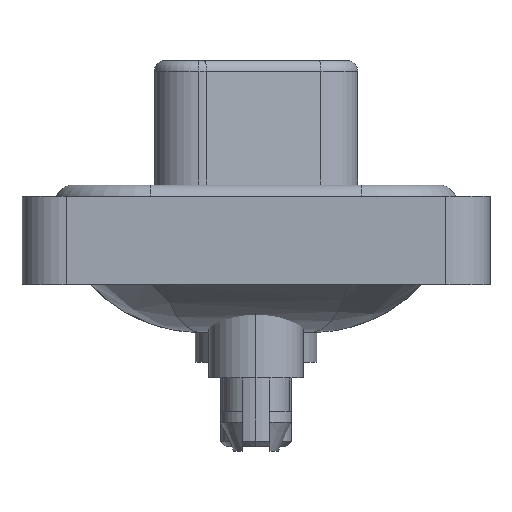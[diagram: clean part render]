
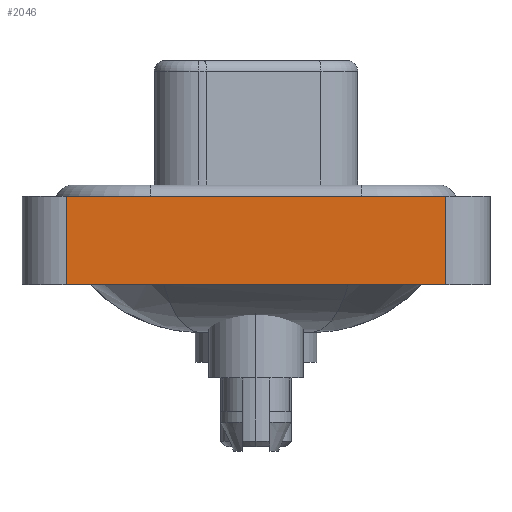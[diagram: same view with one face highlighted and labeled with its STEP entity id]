
A CAD part, left-side view. The second image highlights one B-rep face of the part: STEP entity #2046.
In plain terms, the highlighted planar face has unit normal (-1, 0, 0).
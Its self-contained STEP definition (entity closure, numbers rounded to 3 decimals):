
#1692 = DIRECTION ( 'NONE',  ( 0., -1., 0. ) ) ;
#2046 = ADVANCED_FACE ( 'NONE', ( #7169 ), #2827, .T. ) ;
#2258 = CARTESIAN_POINT ( 'NONE',  ( -7.25, -8.55, -3.6 ) ) ;
#2672 = LINE ( 'NONE', #9816, #17047 ) ;
#2827 = PLANE ( 'NONE',  #12891 ) ;
#2926 = DIRECTION ( 'NONE',  ( -1., 0., 0. ) ) ;
#3456 = VERTEX_POINT ( 'NONE', #10080 ) ;
#3554 = VERTEX_POINT ( 'NONE', #2258 ) ;
#3584 = VECTOR ( 'NONE', #5927, 1000. ) ;
#3691 = VECTOR ( 'NONE', #1692, 1000. ) ;
#3720 = EDGE_CURVE ( 'NONE', #3456, #3554, #6868, .T. ) ;
#4856 = ORIENTED_EDGE ( 'NONE', *, *, #5806, .F. ) ;
#5455 = CARTESIAN_POINT ( 'NONE',  ( -7.25, -8.55, -3.6 ) ) ;
#5572 = DIRECTION ( 'NONE',  ( 0., 0., 1. ) ) ;
#5806 = EDGE_CURVE ( 'NONE', #16466, #14909, #5889, .T. ) ;
#5889 = LINE ( 'NONE', #10043, #3691 ) ;
#5927 = DIRECTION ( 'NONE',  ( 0., 0., 1. ) ) ;
#6868 = LINE ( 'NONE', #5455, #8618 ) ;
#7169 = FACE_OUTER_BOUND ( 'NONE', #17721, .T. ) ;
#7409 = ORIENTED_EDGE ( 'NONE', *, *, #3720, .T. ) ;
#7937 = CARTESIAN_POINT ( 'NONE',  ( -7.25, -8.55, 0.4 ) ) ;
#8618 = VECTOR ( 'NONE', #9496, 1000. ) ;
#9496 = DIRECTION ( 'NONE',  ( 0., -1., 0. ) ) ;
#9816 = CARTESIAN_POINT ( 'NONE',  ( -7.25, -8.55, -3.6 ) ) ;
#9972 = EDGE_CURVE ( 'NONE', #3456, #16466, #15816, .T. ) ;
#10043 = CARTESIAN_POINT ( 'NONE',  ( -7.25, -8.55, 0.4 ) ) ;
#10080 = CARTESIAN_POINT ( 'NONE',  ( -7.25, 8.55, -3.6 ) ) ;
#12891 = AXIS2_PLACEMENT_3D ( 'NONE', #14225, #2926, #14500 ) ;
#13323 = ORIENTED_EDGE ( 'NONE', *, *, #9972, .F. ) ;
#14225 = CARTESIAN_POINT ( 'NONE',  ( -7.25, -8.55, -3.6 ) ) ;
#14500 = DIRECTION ( 'NONE',  ( 0., 0., 1. ) ) ;
#14909 = VERTEX_POINT ( 'NONE', #7937 ) ;
#15436 = CARTESIAN_POINT ( 'NONE',  ( -7.25, 8.55, 0.4 ) ) ;
#15816 = LINE ( 'NONE', #16096, #3584 ) ;
#16064 = EDGE_CURVE ( 'NONE', #3554, #14909, #2672, .T. ) ;
#16096 = CARTESIAN_POINT ( 'NONE',  ( -7.25, 8.55, -3.6 ) ) ;
#16232 = ORIENTED_EDGE ( 'NONE', *, *, #16064, .T. ) ;
#16466 = VERTEX_POINT ( 'NONE', #15436 ) ;
#17047 = VECTOR ( 'NONE', #5572, 1000. ) ;
#17721 = EDGE_LOOP ( 'NONE', ( #16232, #4856, #13323, #7409 ) ) ;
